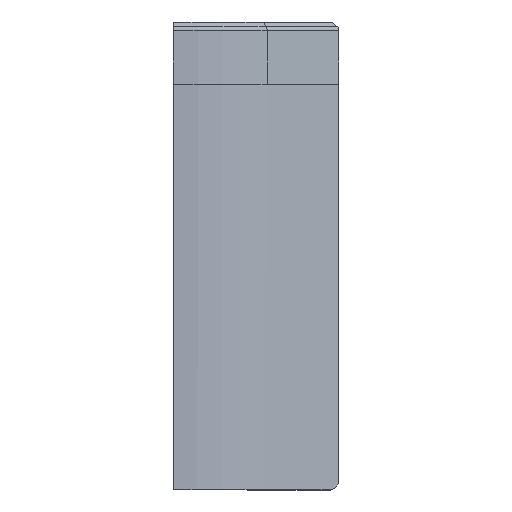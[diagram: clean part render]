
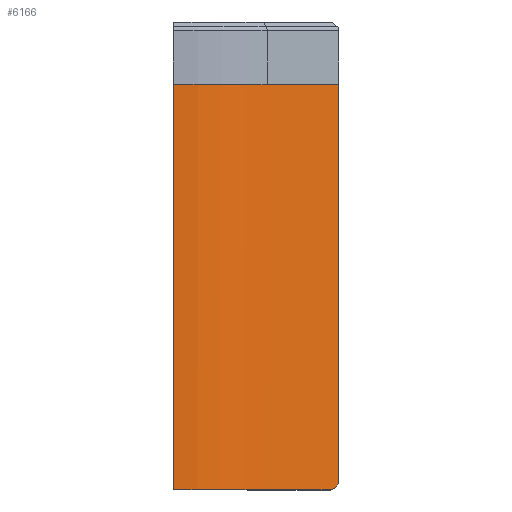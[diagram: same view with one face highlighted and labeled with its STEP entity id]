
A CAD part, front view. The second image highlights one B-rep face of the part: STEP entity #6166.
In plain terms, the highlighted free-form (B-spline) face has degree [3, 1] with [17, 2] control points.
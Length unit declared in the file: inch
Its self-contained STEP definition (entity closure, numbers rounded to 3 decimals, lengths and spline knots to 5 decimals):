
#18 = CARTESIAN_POINT ( 'NONE',  ( 0.37741, -0.539, 0.1 ) ) ;
#128 = CARTESIAN_POINT ( 'NONE',  ( 0.39175, -0.55948, 1.75 ) ) ;
#254 = CARTESIAN_POINT ( 'NONE',  ( 0.40215, -0.52168, 0.1 ) ) ;
#268 = CARTESIAN_POINT ( 'NONE',  ( 0.67121, -0.33352, 0.11321 ) ) ;
#277 = VECTOR ( 'NONE', #11186, 39.37008 ) ;
#477 = FACE_OUTER_BOUND ( 'NONE', #5468, .T. ) ;
#491 = CARTESIAN_POINT ( 'NONE',  ( 0.683, -0.32549, 0.125 ) ) ;
#568 = CARTESIAN_POINT ( 'NONE',  ( 0.65084, -0.34755, 0.1 ) ) ;
#571 = EDGE_CURVE ( 'NONE', #10956, #9532, #5858, .T. ) ;
#823 = CIRCLE ( 'NONE', #3410, 0.683 ) ;
#1103 = CARTESIAN_POINT ( 'NONE',  ( 0.01, -0.68293, 1.75 ) ) ;
#1236 = CARTESIAN_POINT ( 'NONE',  ( -0.20999, -0.66125, 1.75 ) ) ;
#1293 = CARTESIAN_POINT ( 'NONE',  ( -0.46601, -0.50748, 1.75 ) ) ;
#1345 = CARTESIAN_POINT ( 'NONE',  ( 0.683, -0.32503, 0.1 ) ) ;
#1383 = CARTESIAN_POINT ( 'NONE',  ( 0.66, -0.34119, 0.10302 ) ) ;
#1552 = CARTESIAN_POINT ( 'NONE',  ( 0.66532, -0.33754, 0.10732 ) ) ;
#1775 = CARTESIAN_POINT ( 'NONE',  ( 0.01, -0.65793, 0.1 ) ) ;
#1801 = DIRECTION ( 'NONE',  ( 0.819, 0.574, 0. ) ) ;
#1872 = EDGE_CURVE ( 'NONE', #6631, #10978, #7716, .T. ) ;
#1947 = CARTESIAN_POINT ( 'NONE',  ( 0.01, -0.68293, 1.75 ) ) ;
#2403 = CARTESIAN_POINT ( 'NONE',  ( 0.683, -0.35555, 1.75 ) ) ;
#2557 = CARTESIAN_POINT ( 'NONE',  ( -0.53853, -0.4567, 1.75 ) ) ;
#2644 = CARTESIAN_POINT ( 'NONE',  ( 0.01, -0.66787, 0.75603 ) ) ;
#2808 = VERTEX_POINT ( 'NONE', #18 ) ;
#2851 = ORIENTED_EDGE ( 'NONE', *, *, #571, .F. ) ;
#3035 = CARTESIAN_POINT ( 'NONE',  ( 0.45232, -0.48655, 0.1 ) ) ;
#3139 = CARTESIAN_POINT ( 'NONE',  ( 0.53853, -0.4567, 1.75 ) ) ;
#3190 = CARTESIAN_POINT ( 'NONE',  ( -0.683, -0.32503, 0.1 ) ) ;
#3362 = CARTESIAN_POINT ( 'NONE',  ( -0.61055, -0.40628, 1.75 ) ) ;
#3398 = DIRECTION ( 'NONE',  ( 1., 0., 0. ) ) ;
#3410 = AXIS2_PLACEMENT_3D ( 'NONE', #4332, #4390, #3398 ) ;
#3578 = EDGE_CURVE ( 'NONE', #2808, #6551, #10601, .T. ) ;
#3764 = EDGE_CURVE ( 'NONE', #9532, #10862, #823, .T. ) ;
#3784 = CARTESIAN_POINT ( 'NONE',  ( 0., -0.66815, 0.1 ) ) ;
#4011 = CARTESIAN_POINT ( 'NONE',  ( 0.65873, -0.37254, 1.75 ) ) ;
#4078 = CARTESIAN_POINT ( 'NONE',  ( 0.01, -0.65793, 0.1 ) ) ;
#4101 = CARTESIAN_POINT ( 'NONE',  ( 0.65395, -0.34538, 0.10059 ) ) ;
#4121 = CARTESIAN_POINT ( 'NONE',  ( -0.65873, -0.37254, 1.75 ) ) ;
#4332 = CARTESIAN_POINT ( 'NONE',  ( 0., 0., 1.75 ) ) ;
#4380 = CARTESIAN_POINT ( 'NONE',  ( 0.01, -0.67038, 0.92169 ) ) ;
#4390 = DIRECTION ( 'NONE',  ( 0., 0., 1. ) ) ;
#4568 = EDGE_CURVE ( 'NONE', #6551, #11322, #8870, .T. ) ;
#4733 = CARTESIAN_POINT ( 'NONE',  ( 0.683, -0.32549, 0.125 ) ) ;
#4775 = CARTESIAN_POINT ( 'NONE',  ( -0.33553, -0.59885, 1.75 ) ) ;
#4831 = CARTESIAN_POINT ( 'NONE',  ( 0.61055, -0.40628, 1.75 ) ) ;
#4944 = CARTESIAN_POINT ( 'NONE',  ( 0., -0.6939, 1.75 ) ) ;
#5114 = CARTESIAN_POINT ( 'NONE',  ( -0.65753, -0.34286, 0.1 ) ) ;
#5204 = B_SPLINE_CURVE_WITH_KNOTS ( 'NONE', 3,
 ( #9070, #268, #10055, #4733 ),
 .UNSPECIFIED., .F., .F.,
 ( 4, 4 ),
 ( 0.00029, 0.001 ),
 .UNSPECIFIED. ) ;
#5468 = EDGE_LOOP ( 'NONE', ( #2851, #10570, #5766, #7270, #9277, #9475, #11000, #9116 ) ) ;
#5537 = EDGE_CURVE ( 'NONE', #10956, #2808, #6008, .T. ) ;
#5701 = CARTESIAN_POINT ( 'NONE',  ( -0.41677, -0.54197, 1.75 ) ) ;
#5766 = ORIENTED_EDGE ( 'NONE', *, *, #3578, .T. ) ;
#5804 = CARTESIAN_POINT ( 'NONE',  ( 0.41677, -0.54197, 1.75 ) ) ;
#5858 = B_SPLINE_CURVE_WITH_KNOTS ( 'NONE', 3,
 ( #1775, #9875, #10694, #2644, #4380, #8840, #10805, #7918, #10634, #1947 ),
 .UNSPECIFIED., .F., .F.,
 ( 4, 3, 3, 4 ),
 ( 0., 0.01667, 0.02929, 0.04191 ),
 .UNSPECIFIED. ) ;
#6008 = CIRCLE ( 'NONE', #7123, 0.658 ) ;
#6166 = ADVANCED_FACE ( 'NONE', ( #477 ), #7803, .T. ) ;
#6379 = EDGE_CURVE ( 'NONE', #10862, #6631, #7074, .T. ) ;
#6504 = CARTESIAN_POINT ( 'NONE',  ( 0.32181, -0.57794, 0.1 ) ) ;
#6551 = VERTEX_POINT ( 'NONE', #10450 ) ;
#6560 = CARTESIAN_POINT ( 'NONE',  ( -0.32181, -0.57794, 0.1 ) ) ;
#6631 = VERTEX_POINT ( 'NONE', #2403 ) ;
#6667 = CARTESIAN_POINT ( 'NONE',  ( 0.46601, -0.50748, 1.75 ) ) ;
#6941 = VECTOR ( 'NONE', #7247, 39.37008 ) ;
#7074 = LINE ( 'NONE', #128, #6941 ) ;
#7123 = AXIS2_PLACEMENT_3D ( 'NONE', #9304, #8333, #8277 ) ;
#7247 = DIRECTION ( 'NONE',  ( 0.819, 0.574, 0. ) ) ;
#7270 = ORIENTED_EDGE ( 'NONE', *, *, #4568, .T. ) ;
#7317 = CARTESIAN_POINT ( 'NONE',  ( -0.19967, -0.63772, 0.1 ) ) ;
#7483 = VECTOR ( 'NONE', #1801, 39.37008 ) ;
#7546 = CARTESIAN_POINT ( 'NONE',  ( 0.60623, -0.37879, 0.1 ) ) ;
#7599 = CARTESIAN_POINT ( 'NONE',  ( -0.45232, -0.48655, 0.1 ) ) ;
#7716 = LINE ( 'NONE', #10371, #277 ) ;
#7803 = B_SPLINE_SURFACE_WITH_KNOTS ( 'NONE', 3, 1, ( 
 ( #10967, #1345 ),
 ( #4011, #10910 ),
 ( #4831, #7546 ),
 ( #3139, #10095 ),
 ( #6667, #3035 ),
 ( #5804, #254 ),
 ( #8305, #6504 ),
 ( #10202, #9332 ),
 ( #4944, #3784 ),
 ( #1236, #7317 ),
 ( #4775, #6560 ),
 ( #5701, #9221 ),
 ( #1293, #7599 ),
 ( #2557, #11128 ),
 ( #3362, #11303 ),
 ( #4121, #5114 ),
 ( #7834, #3190 ) ),
 .UNSPECIFIED., .F., .F., .F.,
 ( 4, 1, 1, 1, 2, 1, 1, 1, 2, 1, 1, 1, 4 ),
 ( 2, 2 ),
 ( 0., 0.05886, 0.11772, 0.17657, 0.23543, 0.36772, 0.5, 0.63228, 0.76457, 0.82343, 0.88228, 0.94114, 1. ),
 ( 0., 1. ),
 .UNSPECIFIED. ) ;
#7834 = CARTESIAN_POINT ( 'NONE',  ( -0.683, -0.35555, 1.75 ) ) ;
#7918 = CARTESIAN_POINT ( 'NONE',  ( 0.01, -0.67792, 1.41868 ) ) ;
#7942 = EDGE_CURVE ( 'NONE', #11322, #10978, #5204, .T. ) ;
#8277 = DIRECTION ( 'NONE',  ( 1., 0., 0. ) ) ;
#8305 = CARTESIAN_POINT ( 'NONE',  ( 0.33553, -0.59885, 1.75 ) ) ;
#8333 = DIRECTION ( 'NONE',  ( 0., 0., 1. ) ) ;
#8840 = CARTESIAN_POINT ( 'NONE',  ( 0.01, -0.67289, 1.08735 ) ) ;
#8870 = B_SPLINE_CURVE_WITH_KNOTS ( 'NONE', 3,
 ( #10470, #568, #4101, #1383, #10299, #1552 ),
 .UNSPECIFIED., .F., .F.,
 ( 4, 2, 4 ),
 ( 0., 0.00029, 0.00058 ),
 .UNSPECIFIED. ) ;
#9070 = CARTESIAN_POINT ( 'NONE',  ( 0.66532, -0.33754, 0.10732 ) ) ;
#9116 = ORIENTED_EDGE ( 'NONE', *, *, #3764, .F. ) ;
#9221 = CARTESIAN_POINT ( 'NONE',  ( -0.40215, -0.52168, 0.1 ) ) ;
#9277 = ORIENTED_EDGE ( 'NONE', *, *, #7942, .T. ) ;
#9304 = CARTESIAN_POINT ( 'NONE',  ( 0., 0., 0.1 ) ) ;
#9332 = CARTESIAN_POINT ( 'NONE',  ( 0.19967, -0.63772, 0.1 ) ) ;
#9357 = CARTESIAN_POINT ( 'NONE',  ( 0.39175, -0.55948, 1.75 ) ) ;
#9475 = ORIENTED_EDGE ( 'NONE', *, *, #1872, .F. ) ;
#9532 = VERTEX_POINT ( 'NONE', #1103 ) ;
#9725 = CARTESIAN_POINT ( 'NONE',  ( 0.37741, -0.539, 0.1 ) ) ;
#9875 = CARTESIAN_POINT ( 'NONE',  ( 0.01, -0.66124, 0.31868 ) ) ;
#10055 = CARTESIAN_POINT ( 'NONE',  ( 0.67711, -0.32951, 0.11911 ) ) ;
#10095 = CARTESIAN_POINT ( 'NONE',  ( 0.52898, -0.43287, 0.1 ) ) ;
#10202 = CARTESIAN_POINT ( 'NONE',  ( 0.20999, -0.66125, 1.75 ) ) ;
#10299 = CARTESIAN_POINT ( 'NONE',  ( 0.66283, -0.33924, 0.10483 ) ) ;
#10371 = CARTESIAN_POINT ( 'NONE',  ( 0.683, -0.34029, 0.925 ) ) ;
#10450 = CARTESIAN_POINT ( 'NONE',  ( 0.64764, -0.34978, 0.1 ) ) ;
#10470 = CARTESIAN_POINT ( 'NONE',  ( 0.64764, -0.34978, 0.1 ) ) ;
#10570 = ORIENTED_EDGE ( 'NONE', *, *, #5537, .T. ) ;
#10601 = LINE ( 'NONE', #9725, #7483 ) ;
#10634 = CARTESIAN_POINT ( 'NONE',  ( 0.01, -0.68043, 1.58434 ) ) ;
#10694 = CARTESIAN_POINT ( 'NONE',  ( 0.01, -0.66456, 0.53735 ) ) ;
#10805 = CARTESIAN_POINT ( 'NONE',  ( 0.01, -0.67541, 1.25301 ) ) ;
#10862 = VERTEX_POINT ( 'NONE', #9357 ) ;
#10910 = CARTESIAN_POINT ( 'NONE',  ( 0.65753, -0.34286, 0.1 ) ) ;
#10956 = VERTEX_POINT ( 'NONE', #4078 ) ;
#10967 = CARTESIAN_POINT ( 'NONE',  ( 0.683, -0.35555, 1.75 ) ) ;
#10978 = VERTEX_POINT ( 'NONE', #491 ) ;
#11000 = ORIENTED_EDGE ( 'NONE', *, *, #6379, .F. ) ;
#11128 = CARTESIAN_POINT ( 'NONE',  ( -0.52898, -0.43287, 0.1 ) ) ;
#11186 = DIRECTION ( 'NONE',  ( 0., 0.018, -1. ) ) ;
#11303 = CARTESIAN_POINT ( 'NONE',  ( -0.60623, -0.37879, 0.1 ) ) ;
#11322 = VERTEX_POINT ( 'NONE', #11417 ) ;
#11417 = CARTESIAN_POINT ( 'NONE',  ( 0.66532, -0.33754, 0.10732 ) ) ;
